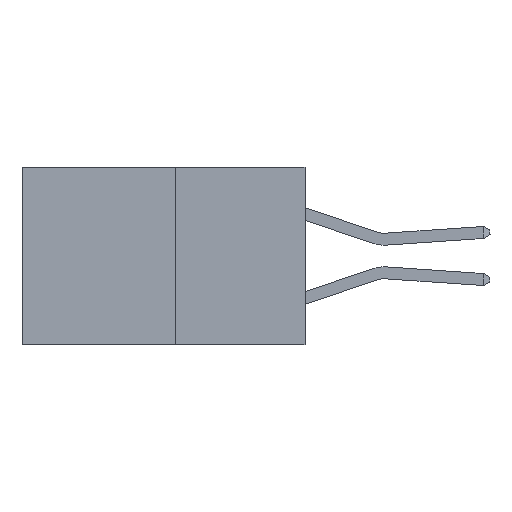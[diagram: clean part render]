
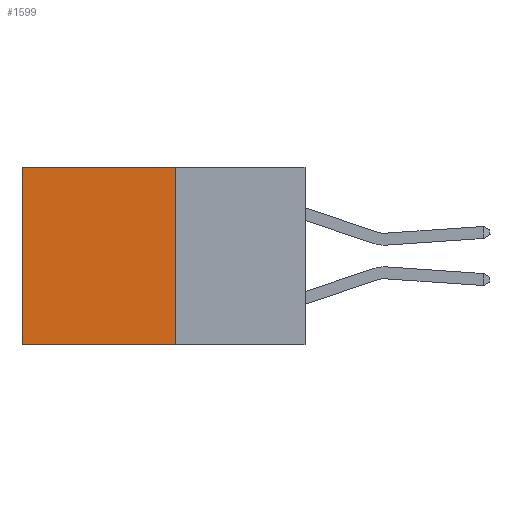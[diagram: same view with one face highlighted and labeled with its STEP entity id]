
A CAD part, left-side view. The second image highlights one B-rep face of the part: STEP entity #1599.
In plain terms, the highlighted planar face has unit normal (-1, 0, 0).
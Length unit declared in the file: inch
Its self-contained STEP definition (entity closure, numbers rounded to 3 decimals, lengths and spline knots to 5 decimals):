
#418 = PLANE ( 'NONE',  #5253 ) ;
#876 = CARTESIAN_POINT ( 'NONE',  ( 0.277, 0.27, -0.37 ) ) ;
#1599 = ADVANCED_FACE ( 'NONE', ( #16315 ), #418, .F. ) ;
#1622 = EDGE_LOOP ( 'NONE', ( #8677, #12022, #16328, #12676 ) ) ;
#2778 = VERTEX_POINT ( 'NONE', #12684 ) ;
#3424 = VECTOR ( 'NONE', #9285, 39.37008 ) ;
#3472 = LINE ( 'NONE', #5321, #6613 ) ;
#3579 = LINE ( 'NONE', #4480, #10583 ) ;
#4480 = CARTESIAN_POINT ( 'NONE',  ( 0.277, 0.27, -0.37 ) ) ;
#5253 = AXIS2_PLACEMENT_3D ( 'NONE', #5949, #6929, #5341 ) ;
#5321 = CARTESIAN_POINT ( 'NONE',  ( 0.277, 0.27, -0.37 ) ) ;
#5341 = DIRECTION ( 'NONE',  ( 0., 0., -1. ) ) ;
#5392 = CARTESIAN_POINT ( 'NONE',  ( 0.277, 0.59, -0.37 ) ) ;
#5949 = CARTESIAN_POINT ( 'NONE',  ( 0.277, 0.27, -0.37 ) ) ;
#6613 = VECTOR ( 'NONE', #6623, 39.37008 ) ;
#6623 = DIRECTION ( 'NONE',  ( 0., 0., -1. ) ) ;
#6658 = VECTOR ( 'NONE', #13815, 39.37008 ) ;
#6929 = DIRECTION ( 'NONE',  ( 1., 0., 0. ) ) ;
#6962 = LINE ( 'NONE', #5392, #3424 ) ;
#8677 = ORIENTED_EDGE ( 'NONE', *, *, #12817, .T. ) ;
#9285 = DIRECTION ( 'NONE',  ( 0., 0., -1. ) ) ;
#10583 = VECTOR ( 'NONE', #12363, 39.37008 ) ;
#11134 = CARTESIAN_POINT ( 'NONE',  ( 0.277, 0.59, 0. ) ) ;
#11165 = VERTEX_POINT ( 'NONE', #11134 ) ;
#11553 = EDGE_CURVE ( 'NONE', #13684, #12107, #3472, .T. ) ;
#12022 = ORIENTED_EDGE ( 'NONE', *, *, #14389, .F. ) ;
#12107 = VERTEX_POINT ( 'NONE', #876 ) ;
#12363 = DIRECTION ( 'NONE',  ( 0., 1., 0. ) ) ;
#12676 = ORIENTED_EDGE ( 'NONE', *, *, #15738, .T. ) ;
#12684 = CARTESIAN_POINT ( 'NONE',  ( 0.277, 0.59, -0.37 ) ) ;
#12817 = EDGE_CURVE ( 'NONE', #11165, #2778, #6962, .T. ) ;
#13684 = VERTEX_POINT ( 'NONE', #14877 ) ;
#13815 = DIRECTION ( 'NONE',  ( 0., 1., 0. ) ) ;
#14389 = EDGE_CURVE ( 'NONE', #12107, #2778, #3579, .T. ) ;
#14877 = CARTESIAN_POINT ( 'NONE',  ( 0.277, 0.27, 0. ) ) ;
#15074 = CARTESIAN_POINT ( 'NONE',  ( 0.277, 0.27, 0. ) ) ;
#15738 = EDGE_CURVE ( 'NONE', #13684, #11165, #17091, .T. ) ;
#16315 = FACE_OUTER_BOUND ( 'NONE', #1622, .T. ) ;
#16328 = ORIENTED_EDGE ( 'NONE', *, *, #11553, .F. ) ;
#17091 = LINE ( 'NONE', #15074, #6658 ) ;
